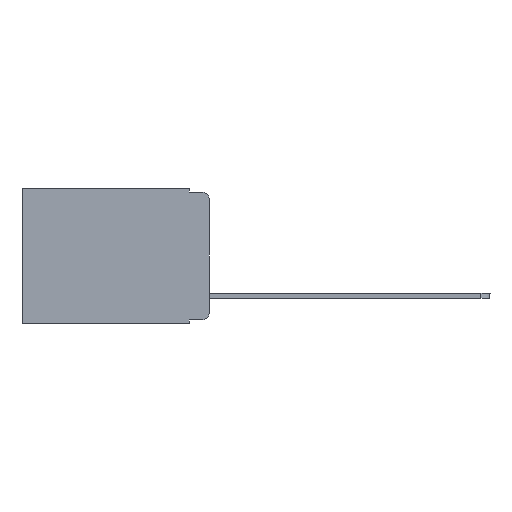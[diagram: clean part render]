
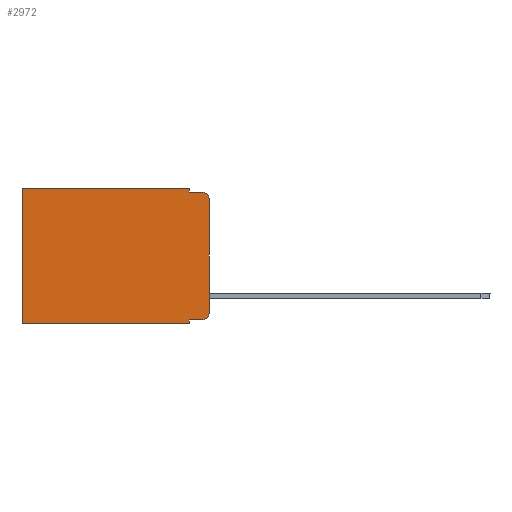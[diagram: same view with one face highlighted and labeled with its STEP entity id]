
A CAD part, left-side view. The second image highlights one B-rep face of the part: STEP entity #2972.
In plain terms, the highlighted planar face has unit normal (-1, 0, 0).
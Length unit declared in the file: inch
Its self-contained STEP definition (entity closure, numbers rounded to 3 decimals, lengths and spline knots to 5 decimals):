
#441 = VECTOR ( 'NONE', #3544, 39.37008 ) ;
#466 = CARTESIAN_POINT ( 'NONE',  ( 0.298, 0.051, 0. ) ) ;
#697 = VECTOR ( 'NONE', #20423, 39.37008 ) ;
#1054 = ORIENTED_EDGE ( 'NONE', *, *, #13312, .F. ) ;
#1276 = ORIENTED_EDGE ( 'NONE', *, *, #2161, .T. ) ;
#1459 = DIRECTION ( 'NONE',  ( 0., 1., 0. ) ) ;
#1724 = ORIENTED_EDGE ( 'NONE', *, *, #15315, .T. ) ;
#1826 = CARTESIAN_POINT ( 'NONE',  ( 0.298, 0.051, -0.333 ) ) ;
#1909 = DIRECTION ( 'NONE',  ( 0., 0., -1. ) ) ;
#2161 = EDGE_CURVE ( 'NONE', #16751, #24505, #3697, .T. ) ;
#2474 = LINE ( 'NONE', #466, #10606 ) ;
#2972 = ADVANCED_FACE ( 'NONE', ( #12759 ), #7139, .F. ) ;
#3157 = DIRECTION ( 'NONE',  ( 0., 0., -1. ) ) ;
#3544 = DIRECTION ( 'NONE',  ( 0., 0., -1. ) ) ;
#3617 = EDGE_CURVE ( 'NONE', #9934, #22794, #2474, .T. ) ;
#3697 = LINE ( 'NONE', #1826, #697 ) ;
#4254 = VERTEX_POINT ( 'NONE', #9982 ) ;
#4496 = EDGE_CURVE ( 'NONE', #9934, #9871, #22299, .T. ) ;
#4759 = DIRECTION ( 'NONE',  ( -1., 0., 0. ) ) ;
#4870 = CARTESIAN_POINT ( 'NONE',  ( 0.298, 0.473, 0. ) ) ;
#5219 = CARTESIAN_POINT ( 'NONE',  ( 0.298, 0.02, -0.01 ) ) ;
#5400 = CARTESIAN_POINT ( 'NONE',  ( 0.298, 0.473, 0. ) ) ;
#5504 = CARTESIAN_POINT ( 'NONE',  ( 0.298, 0., 0. ) ) ;
#5906 = DIRECTION ( 'NONE',  ( 0., 0., -1. ) ) ;
#6187 = LINE ( 'NONE', #8436, #7820 ) ;
#6930 = DIRECTION ( 'NONE',  ( 0., 0., -1. ) ) ;
#7139 = PLANE ( 'NONE',  #8399 ) ;
#7736 = CARTESIAN_POINT ( 'NONE',  ( 0.298, 0.051, -0.343 ) ) ;
#7820 = VECTOR ( 'NONE', #19911, 39.37008 ) ;
#8166 = CARTESIAN_POINT ( 'NONE',  ( 0.298, 0.02, -0.03 ) ) ;
#8399 = AXIS2_PLACEMENT_3D ( 'NONE', #5504, #13006, #3157 ) ;
#8436 = CARTESIAN_POINT ( 'NONE',  ( 0.298, 0.051, -0.01 ) ) ;
#8627 = DIRECTION ( 'NONE',  ( 0., 0., -1. ) ) ;
#8824 = EDGE_CURVE ( 'NONE', #22794, #24686, #6187, .T. ) ;
#8893 = VECTOR ( 'NONE', #1909, 39.37008 ) ;
#8921 = CARTESIAN_POINT ( 'NONE',  ( 0.298, 0.473, -0.343 ) ) ;
#8956 = VERTEX_POINT ( 'NONE', #8921 ) ;
#9297 = VERTEX_POINT ( 'NONE', #10155 ) ;
#9871 = VERTEX_POINT ( 'NONE', #4870 ) ;
#9906 = EDGE_CURVE ( 'NONE', #12638, #8956, #18611, .T. ) ;
#9934 = VERTEX_POINT ( 'NONE', #16986 ) ;
#9982 = CARTESIAN_POINT ( 'NONE',  ( 0.298, 0., -0.313 ) ) ;
#10155 = CARTESIAN_POINT ( 'NONE',  ( 0.298, 0., -0.03 ) ) ;
#10459 = EDGE_LOOP ( 'NONE', ( #17937, #22886, #15964, #24535, #13657, #1724, #23138, #1054, #1276, #23473 ) ) ;
#10606 = VECTOR ( 'NONE', #15950, 39.37008 ) ;
#10802 = LINE ( 'NONE', #11066, #13517 ) ;
#10817 = CARTESIAN_POINT ( 'NONE',  ( 0.298, 0.051, -0.333 ) ) ;
#11066 = CARTESIAN_POINT ( 'NONE',  ( 0.298, 0.051, 0. ) ) ;
#12263 = VECTOR ( 'NONE', #24481, 39.37008 ) ;
#12280 = CIRCLE ( 'NONE', #22239, 0.02 ) ;
#12326 = EDGE_CURVE ( 'NONE', #24505, #4254, #12280, .T. ) ;
#12360 = CARTESIAN_POINT ( 'NONE',  ( 0.298, 0.02, -0.333 ) ) ;
#12638 = VERTEX_POINT ( 'NONE', #7736 ) ;
#12759 = FACE_OUTER_BOUND ( 'NONE', #10459, .T. ) ;
#13006 = DIRECTION ( 'NONE',  ( 1., 0., 0. ) ) ;
#13239 = CIRCLE ( 'NONE', #19993, 0.02 ) ;
#13312 = EDGE_CURVE ( 'NONE', #16751, #12638, #10802, .T. ) ;
#13517 = VECTOR ( 'NONE', #6930, 39.37008 ) ;
#13657 = ORIENTED_EDGE ( 'NONE', *, *, #4496, .T. ) ;
#14504 = CARTESIAN_POINT ( 'NONE',  ( 0.298, 0.02, -0.313 ) ) ;
#15148 = CARTESIAN_POINT ( 'NONE',  ( 0.298, 0., 0. ) ) ;
#15315 = EDGE_CURVE ( 'NONE', #9871, #8956, #22509, .T. ) ;
#15950 = DIRECTION ( 'NONE',  ( 0., 0., -1. ) ) ;
#15964 = ORIENTED_EDGE ( 'NONE', *, *, #8824, .F. ) ;
#16434 = VECTOR ( 'NONE', #1459, 39.37008 ) ;
#16617 = CARTESIAN_POINT ( 'NONE',  ( 0.298, 0., -0.343 ) ) ;
#16751 = VERTEX_POINT ( 'NONE', #10817 ) ;
#16986 = CARTESIAN_POINT ( 'NONE',  ( 0.298, 0.051, 0. ) ) ;
#17937 = ORIENTED_EDGE ( 'NONE', *, *, #22563, .F. ) ;
#18444 = CARTESIAN_POINT ( 'NONE',  ( 0.298, 0., 0. ) ) ;
#18611 = LINE ( 'NONE', #16617, #12263 ) ;
#19656 = EDGE_CURVE ( 'NONE', #9297, #24686, #13239, .T. ) ;
#19911 = DIRECTION ( 'NONE',  ( 0., -1., 0. ) ) ;
#19993 = AXIS2_PLACEMENT_3D ( 'NONE', #8166, #23028, #5906 ) ;
#20423 = DIRECTION ( 'NONE',  ( 0., -1., 0. ) ) ;
#22090 = CARTESIAN_POINT ( 'NONE',  ( 0.298, 0.051, -0.01 ) ) ;
#22239 = AXIS2_PLACEMENT_3D ( 'NONE', #14504, #4759, #8627 ) ;
#22299 = LINE ( 'NONE', #18444, #16434 ) ;
#22509 = LINE ( 'NONE', #5400, #441 ) ;
#22563 = EDGE_CURVE ( 'NONE', #9297, #4254, #24637, .T. ) ;
#22794 = VERTEX_POINT ( 'NONE', #22090 ) ;
#22886 = ORIENTED_EDGE ( 'NONE', *, *, #19656, .T. ) ;
#23028 = DIRECTION ( 'NONE',  ( -1., 0., 0. ) ) ;
#23138 = ORIENTED_EDGE ( 'NONE', *, *, #9906, .F. ) ;
#23473 = ORIENTED_EDGE ( 'NONE', *, *, #12326, .T. ) ;
#24481 = DIRECTION ( 'NONE',  ( 0., 1., 0. ) ) ;
#24505 = VERTEX_POINT ( 'NONE', #12360 ) ;
#24535 = ORIENTED_EDGE ( 'NONE', *, *, #3617, .F. ) ;
#24637 = LINE ( 'NONE', #15148, #8893 ) ;
#24686 = VERTEX_POINT ( 'NONE', #5219 ) ;
